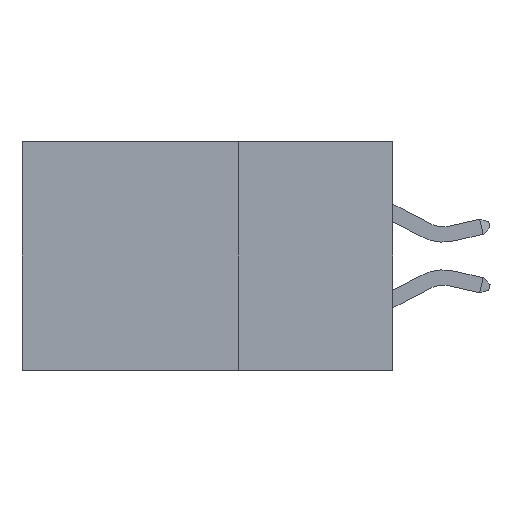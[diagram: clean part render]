
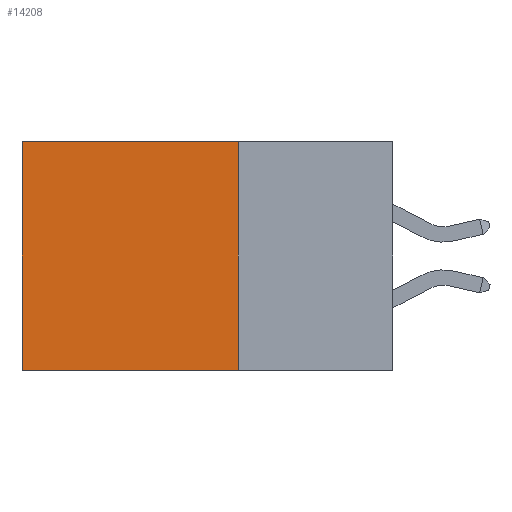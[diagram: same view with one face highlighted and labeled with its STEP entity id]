
A CAD part, left-side view. The second image highlights one B-rep face of the part: STEP entity #14208.
In plain terms, the highlighted planar face has unit normal (-1, 0, 0).
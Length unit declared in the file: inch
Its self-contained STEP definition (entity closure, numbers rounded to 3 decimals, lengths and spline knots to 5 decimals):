
#1024 = ORIENTED_EDGE ( 'NONE', *, *, #9620, .T. ) ;
#2011 = EDGE_CURVE ( 'NONE', #17123, #14223, #15689, .T. ) ;
#3470 = AXIS2_PLACEMENT_3D ( 'NONE', #20498, #18626, #24187 ) ;
#5059 = ORIENTED_EDGE ( 'NONE', *, *, #13824, .F. ) ;
#6302 = CARTESIAN_POINT ( 'NONE',  ( 0.2875, 0.6, 0. ) ) ;
#6657 = DIRECTION ( 'NONE',  ( 0., 0., -1. ) ) ;
#6751 = LINE ( 'NONE', #17393, #16497 ) ;
#7834 = VECTOR ( 'NONE', #22839, 39.37008 ) ;
#9620 = EDGE_CURVE ( 'NONE', #13658, #14223, #22780, .T. ) ;
#10820 = CARTESIAN_POINT ( 'NONE',  ( 0.2875, 0.25, 0. ) ) ;
#11687 = VECTOR ( 'NONE', #6657, 39.37008 ) ;
#12240 = ORIENTED_EDGE ( 'NONE', *, *, #17033, .T. ) ;
#12455 = DIRECTION ( 'NONE',  ( 0., 1., 0. ) ) ;
#13658 = VERTEX_POINT ( 'NONE', #16184 ) ;
#13824 = EDGE_CURVE ( 'NONE', #20282, #17123, #18223, .T. ) ;
#14178 = FACE_OUTER_BOUND ( 'NONE', #24075, .T. ) ;
#14208 = ADVANCED_FACE ( 'NONE', ( #14178 ), #22573, .F. ) ;
#14223 = VERTEX_POINT ( 'NONE', #16614 ) ;
#14477 = VECTOR ( 'NONE', #12455, 39.37008 ) ;
#15499 = CARTESIAN_POINT ( 'NONE',  ( 0.2875, 0.25, 0. ) ) ;
#15689 = LINE ( 'NONE', #24423, #14477 ) ;
#16184 = CARTESIAN_POINT ( 'NONE',  ( 0.2875, 0.6, 0. ) ) ;
#16497 = VECTOR ( 'NONE', #17472, 39.37008 ) ;
#16614 = CARTESIAN_POINT ( 'NONE',  ( 0.2875, 0.6, -0.37 ) ) ;
#17033 = EDGE_CURVE ( 'NONE', #20282, #13658, #6751, .T. ) ;
#17123 = VERTEX_POINT ( 'NONE', #23509 ) ;
#17393 = CARTESIAN_POINT ( 'NONE',  ( 0.2875, 0.25, 0. ) ) ;
#17472 = DIRECTION ( 'NONE',  ( 0., 1., 0. ) ) ;
#18223 = LINE ( 'NONE', #10820, #7834 ) ;
#18626 = DIRECTION ( 'NONE',  ( 1., 0., 0. ) ) ;
#20282 = VERTEX_POINT ( 'NONE', #15499 ) ;
#20498 = CARTESIAN_POINT ( 'NONE',  ( 0.2875, 0.25, 0. ) ) ;
#22573 = PLANE ( 'NONE',  #3470 ) ;
#22780 = LINE ( 'NONE', #6302, #11687 ) ;
#22839 = DIRECTION ( 'NONE',  ( 0., 0., -1. ) ) ;
#23509 = CARTESIAN_POINT ( 'NONE',  ( 0.2875, 0.25, -0.37 ) ) ;
#24075 = EDGE_LOOP ( 'NONE', ( #1024, #24327, #5059, #12240 ) ) ;
#24187 = DIRECTION ( 'NONE',  ( 0., 0., -1. ) ) ;
#24327 = ORIENTED_EDGE ( 'NONE', *, *, #2011, .F. ) ;
#24423 = CARTESIAN_POINT ( 'NONE',  ( 0.2875, 0.25, -0.37 ) ) ;
